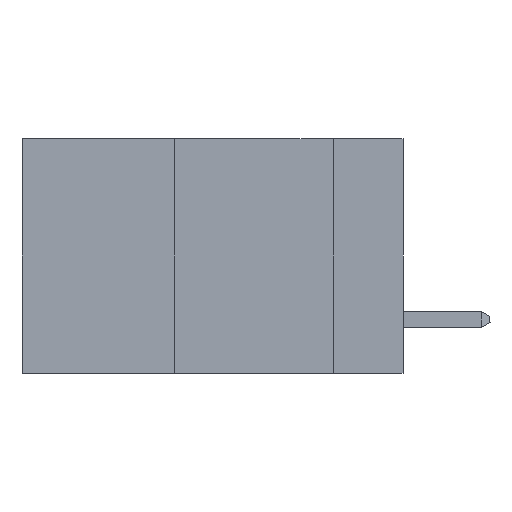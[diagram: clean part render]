
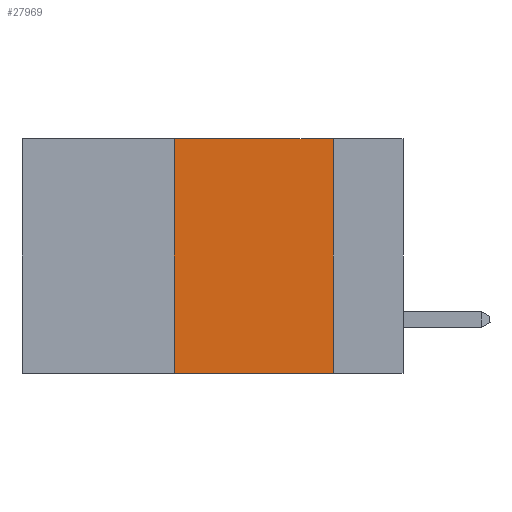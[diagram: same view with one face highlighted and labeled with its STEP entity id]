
A CAD part, left-side view. The second image highlights one B-rep face of the part: STEP entity #27969.
In plain terms, the highlighted planar face has unit normal (-1, 0, 0).
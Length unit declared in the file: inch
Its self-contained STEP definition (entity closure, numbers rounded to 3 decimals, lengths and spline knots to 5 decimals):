
#519 = DIRECTION ( 'NONE',  ( 0., -1., 0. ) ) ;
#1111 = FACE_OUTER_BOUND ( 'NONE', #24469, .T. ) ;
#2261 = ORIENTED_EDGE ( 'NONE', *, *, #6593, .T. ) ;
#3029 = VERTEX_POINT ( 'NONE', #20228 ) ;
#3097 = LINE ( 'NONE', #7089, #14080 ) ;
#3216 = CARTESIAN_POINT ( 'NONE',  ( 0., 0.6, 0. ) ) ;
#4667 = ORIENTED_EDGE ( 'NONE', *, *, #10841, .F. ) ;
#4824 = VECTOR ( 'NONE', #6352, 39.37008 ) ;
#5603 = VECTOR ( 'NONE', #13988, 39.37008 ) ;
#5934 = DIRECTION ( 'NONE',  ( 0., 0., -1. ) ) ;
#5993 = CARTESIAN_POINT ( 'NONE',  ( 0., 0.36, 0. ) ) ;
#6027 = LINE ( 'NONE', #19634, #5603 ) ;
#6352 = DIRECTION ( 'NONE',  ( 0., 0., 1. ) ) ;
#6593 = EDGE_CURVE ( 'NONE', #32879, #3029, #29155, .T. ) ;
#7089 = CARTESIAN_POINT ( 'NONE',  ( 0., 0.6, 0. ) ) ;
#8886 = CARTESIAN_POINT ( 'NONE',  ( 0., 0.11, 0. ) ) ;
#10051 = AXIS2_PLACEMENT_3D ( 'NONE', #3216, #23728, #5934 ) ;
#10841 = EDGE_CURVE ( 'NONE', #26770, #3029, #6027, .T. ) ;
#13386 = CARTESIAN_POINT ( 'NONE',  ( 0., 0.6, -0.37 ) ) ;
#13988 = DIRECTION ( 'NONE',  ( 0., 0., -1. ) ) ;
#14080 = VECTOR ( 'NONE', #15247, 39.37008 ) ;
#15247 = DIRECTION ( 'NONE',  ( 0., -1., 0. ) ) ;
#15372 = VECTOR ( 'NONE', #519, 39.37008 ) ;
#16656 = ORIENTED_EDGE ( 'NONE', *, *, #27286, .F. ) ;
#19634 = CARTESIAN_POINT ( 'NONE',  ( 0., 0.11, 0. ) ) ;
#20228 = CARTESIAN_POINT ( 'NONE',  ( 0., 0.11, -0.37 ) ) ;
#20443 = VERTEX_POINT ( 'NONE', #5993 ) ;
#22474 = EDGE_CURVE ( 'NONE', #20443, #26770, #3097, .T. ) ;
#22643 = LINE ( 'NONE', #27022, #4824 ) ;
#23728 = DIRECTION ( 'NONE',  ( 1., 0., 0. ) ) ;
#24469 = EDGE_LOOP ( 'NONE', ( #4667, #27840, #16656, #2261 ) ) ;
#26770 = VERTEX_POINT ( 'NONE', #8886 ) ;
#27022 = CARTESIAN_POINT ( 'NONE',  ( 0., 0.36, 0. ) ) ;
#27286 = EDGE_CURVE ( 'NONE', #32879, #20443, #22643, .T. ) ;
#27840 = ORIENTED_EDGE ( 'NONE', *, *, #22474, .F. ) ;
#27969 = ADVANCED_FACE ( 'NONE', ( #1111 ), #31778, .F. ) ;
#29014 = CARTESIAN_POINT ( 'NONE',  ( 0., 0.36, -0.37 ) ) ;
#29155 = LINE ( 'NONE', #13386, #15372 ) ;
#31778 = PLANE ( 'NONE',  #10051 ) ;
#32879 = VERTEX_POINT ( 'NONE', #29014 ) ;
